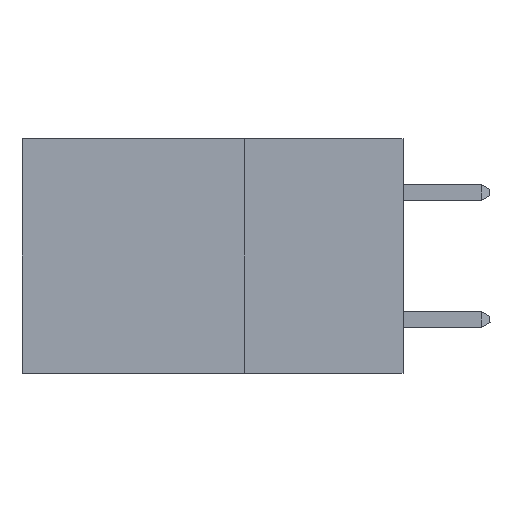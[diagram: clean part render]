
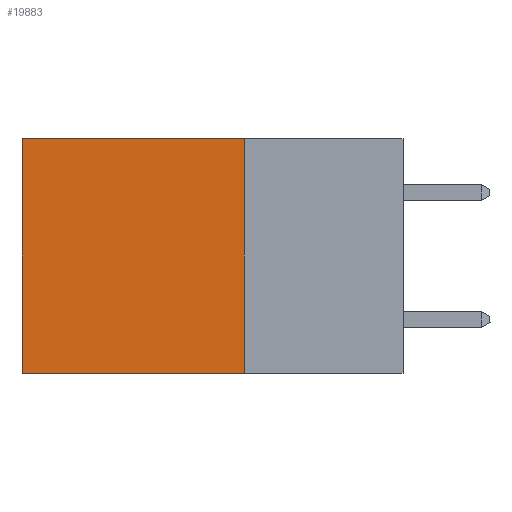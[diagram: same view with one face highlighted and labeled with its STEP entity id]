
A CAD part, left-side view. The second image highlights one B-rep face of the part: STEP entity #19883.
In plain terms, the highlighted planar face has unit normal (-1, 0, 0).
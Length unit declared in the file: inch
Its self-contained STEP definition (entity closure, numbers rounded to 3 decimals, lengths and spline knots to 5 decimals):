
#15 = LINE ( 'NONE', #12571, #22839 ) ;
#1331 = VERTEX_POINT ( 'NONE', #12472 ) ;
#1379 = DIRECTION ( 'NONE',  ( 0., 0., -1. ) ) ;
#1806 = LINE ( 'NONE', #9744, #22558 ) ;
#3451 = VERTEX_POINT ( 'NONE', #23239 ) ;
#3769 = EDGE_CURVE ( 'NONE', #1331, #7499, #15, .T. ) ;
#4680 = ORIENTED_EDGE ( 'NONE', *, *, #3769, .T. ) ;
#5739 = DIRECTION ( 'NONE',  ( 0., 1., 0. ) ) ;
#6155 = LINE ( 'NONE', #20664, #10866 ) ;
#6749 = CARTESIAN_POINT ( 'NONE',  ( 0.2875, 0.6, 0. ) ) ;
#7049 = EDGE_CURVE ( 'NONE', #3451, #13185, #6155, .T. ) ;
#7499 = VERTEX_POINT ( 'NONE', #6749 ) ;
#7749 = EDGE_CURVE ( 'NONE', #7499, #13185, #1806, .T. ) ;
#8425 = ORIENTED_EDGE ( 'NONE', *, *, #16780, .F. ) ;
#8970 = DIRECTION ( 'NONE',  ( 0., 0., -1. ) ) ;
#9694 = ORIENTED_EDGE ( 'NONE', *, *, #7049, .F. ) ;
#9744 = CARTESIAN_POINT ( 'NONE',  ( 0.2875, 0.6, 0. ) ) ;
#10071 = FACE_OUTER_BOUND ( 'NONE', #24184, .T. ) ;
#10866 = VECTOR ( 'NONE', #5739, 39.37008 ) ;
#12472 = CARTESIAN_POINT ( 'NONE',  ( 0.2875, 0.25, 0. ) ) ;
#12571 = CARTESIAN_POINT ( 'NONE',  ( 0.2875, 0.25, 0. ) ) ;
#12742 = DIRECTION ( 'NONE',  ( 1., 0., 0. ) ) ;
#13185 = VERTEX_POINT ( 'NONE', #23054 ) ;
#14484 = CARTESIAN_POINT ( 'NONE',  ( 0.2875, 0.25, 0. ) ) ;
#16459 = PLANE ( 'NONE',  #23832 ) ;
#16749 = ORIENTED_EDGE ( 'NONE', *, *, #7749, .T. ) ;
#16780 = EDGE_CURVE ( 'NONE', #1331, #3451, #21202, .T. ) ;
#17200 = DIRECTION ( 'NONE',  ( 0., 0., -1. ) ) ;
#19883 = ADVANCED_FACE ( 'NONE', ( #10071 ), #16459, .F. ) ;
#20395 = CARTESIAN_POINT ( 'NONE',  ( 0.2875, 0.25, 0. ) ) ;
#20664 = CARTESIAN_POINT ( 'NONE',  ( 0.2875, 0.25, -0.37 ) ) ;
#21202 = LINE ( 'NONE', #20395, #21784 ) ;
#21784 = VECTOR ( 'NONE', #8970, 39.37008 ) ;
#22558 = VECTOR ( 'NONE', #17200, 39.37008 ) ;
#22839 = VECTOR ( 'NONE', #23731, 39.37008 ) ;
#23054 = CARTESIAN_POINT ( 'NONE',  ( 0.2875, 0.6, -0.37 ) ) ;
#23239 = CARTESIAN_POINT ( 'NONE',  ( 0.2875, 0.25, -0.37 ) ) ;
#23731 = DIRECTION ( 'NONE',  ( 0., 1., 0. ) ) ;
#23832 = AXIS2_PLACEMENT_3D ( 'NONE', #14484, #12742, #1379 ) ;
#24184 = EDGE_LOOP ( 'NONE', ( #16749, #9694, #8425, #4680 ) ) ;
